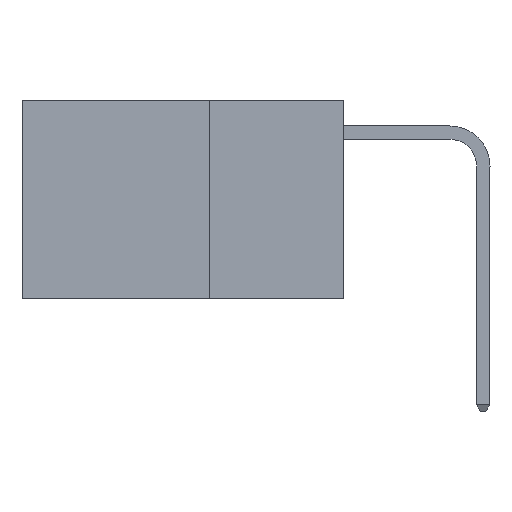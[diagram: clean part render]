
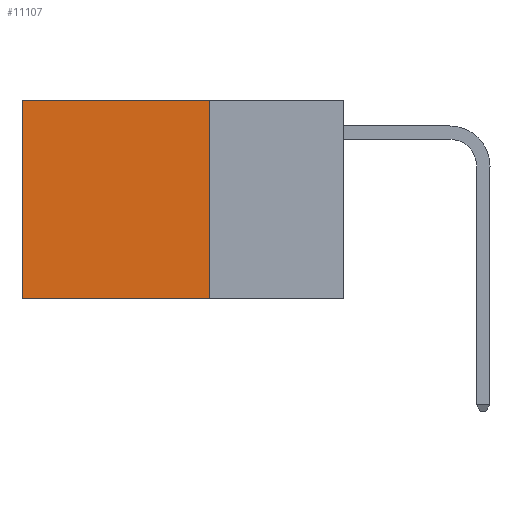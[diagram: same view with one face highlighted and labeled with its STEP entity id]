
A CAD part, left-side view. The second image highlights one B-rep face of the part: STEP entity #11107.
In plain terms, the highlighted planar face has unit normal (-1, 0, 0).
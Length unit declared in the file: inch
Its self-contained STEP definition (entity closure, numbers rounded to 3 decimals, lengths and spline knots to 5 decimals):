
#43 = ORIENTED_EDGE ( 'NONE', *, *, #17475, .T. ) ;
#589 = DIRECTION ( 'NONE',  ( 1., 0., 0. ) ) ;
#680 = CARTESIAN_POINT ( 'NONE',  ( 0.2625, 0.25, 0. ) ) ;
#726 = DIRECTION ( 'NONE',  ( 0., 0., -1. ) ) ;
#1255 = CARTESIAN_POINT ( 'NONE',  ( 0.2625, 0.6, -0.37 ) ) ;
#1630 = CARTESIAN_POINT ( 'NONE',  ( 0.2625, 0.25, 0. ) ) ;
#1702 = ORIENTED_EDGE ( 'NONE', *, *, #11152, .T. ) ;
#1989 = CARTESIAN_POINT ( 'NONE',  ( 0.2625, 0.25, 0. ) ) ;
#2592 = CARTESIAN_POINT ( 'NONE',  ( 0.2625, 0.25, -0.37 ) ) ;
#2652 = DIRECTION ( 'NONE',  ( 0., 1., 0. ) ) ;
#3862 = VECTOR ( 'NONE', #17762, 39.37008 ) ;
#4070 = EDGE_CURVE ( 'NONE', #7578, #8589, #10263, .T. ) ;
#6639 = VECTOR ( 'NONE', #11222, 39.37008 ) ;
#7158 = VECTOR ( 'NONE', #726, 39.37008 ) ;
#7578 = VERTEX_POINT ( 'NONE', #14322 ) ;
#7991 = LINE ( 'NONE', #680, #3862 ) ;
#8336 = PLANE ( 'NONE',  #13168 ) ;
#8589 = VERTEX_POINT ( 'NONE', #1255 ) ;
#8984 = VERTEX_POINT ( 'NONE', #17708 ) ;
#10263 = LINE ( 'NONE', #2592, #13463 ) ;
#10670 = ORIENTED_EDGE ( 'NONE', *, *, #4070, .F. ) ;
#10673 = LINE ( 'NONE', #1989, #6639 ) ;
#11107 = ADVANCED_FACE ( 'NONE', ( #12207 ), #8336, .F. ) ;
#11152 = EDGE_CURVE ( 'NONE', #8984, #8589, #15382, .T. ) ;
#11222 = DIRECTION ( 'NONE',  ( 0., 1., 0. ) ) ;
#11391 = DIRECTION ( 'NONE',  ( 0., 0., -1. ) ) ;
#12207 = FACE_OUTER_BOUND ( 'NONE', #14841, .T. ) ;
#12811 = VERTEX_POINT ( 'NONE', #1630 ) ;
#13168 = AXIS2_PLACEMENT_3D ( 'NONE', #19138, #589, #11391 ) ;
#13463 = VECTOR ( 'NONE', #2652, 39.37008 ) ;
#13521 = ORIENTED_EDGE ( 'NONE', *, *, #19246, .F. ) ;
#14322 = CARTESIAN_POINT ( 'NONE',  ( 0.2625, 0.25, -0.37 ) ) ;
#14841 = EDGE_LOOP ( 'NONE', ( #1702, #10670, #13521, #43 ) ) ;
#15382 = LINE ( 'NONE', #19203, #7158 ) ;
#17475 = EDGE_CURVE ( 'NONE', #12811, #8984, #10673, .T. ) ;
#17708 = CARTESIAN_POINT ( 'NONE',  ( 0.2625, 0.6, 0. ) ) ;
#17762 = DIRECTION ( 'NONE',  ( 0., 0., -1. ) ) ;
#19138 = CARTESIAN_POINT ( 'NONE',  ( 0.2625, 0.25, 0. ) ) ;
#19203 = CARTESIAN_POINT ( 'NONE',  ( 0.2625, 0.6, 0. ) ) ;
#19246 = EDGE_CURVE ( 'NONE', #12811, #7578, #7991, .T. ) ;
